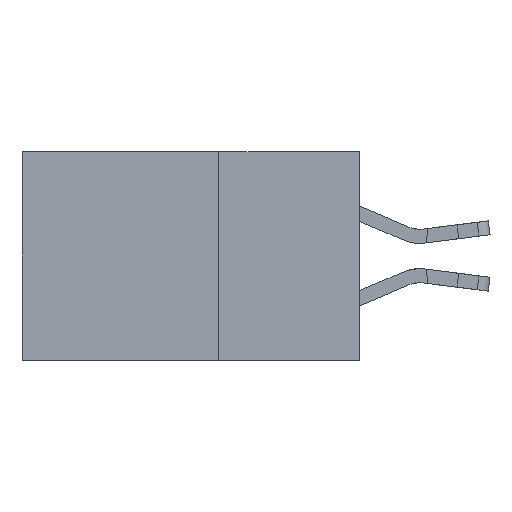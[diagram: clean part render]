
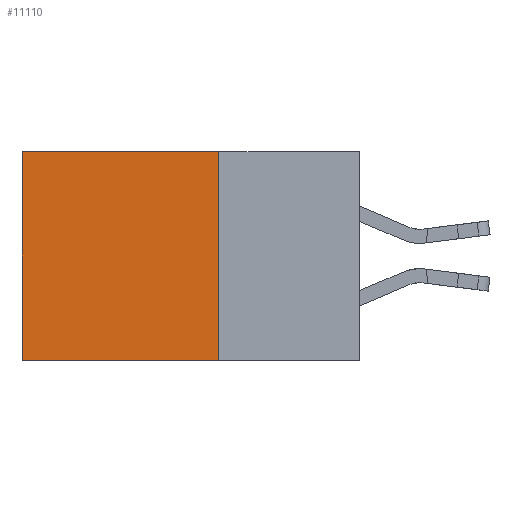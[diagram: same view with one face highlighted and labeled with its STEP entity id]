
A CAD part, left-side view. The second image highlights one B-rep face of the part: STEP entity #11110.
In plain terms, the highlighted planar face has unit normal (-1, 0, 0).
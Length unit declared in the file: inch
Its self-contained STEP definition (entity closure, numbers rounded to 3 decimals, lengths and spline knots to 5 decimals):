
#497 = CARTESIAN_POINT ( 'NONE',  ( 0.2875, 0.6, 0. ) ) ;
#4313 = LINE ( 'NONE', #4656, #7326 ) ;
#4656 = CARTESIAN_POINT ( 'NONE',  ( 0.2875, 0.25, 0. ) ) ;
#5316 = VECTOR ( 'NONE', #18281, 39.37008 ) ;
#6180 = CARTESIAN_POINT ( 'NONE',  ( 0.2875, 0.25, 0. ) ) ;
#7059 = EDGE_CURVE ( 'NONE', #25627, #17850, #20991, .T. ) ;
#7195 = DIRECTION ( 'NONE',  ( 0., 0., -1. ) ) ;
#7263 = CARTESIAN_POINT ( 'NONE',  ( 0.2875, 0.25, -0.37 ) ) ;
#7326 = VECTOR ( 'NONE', #7195, 39.37008 ) ;
#7953 = EDGE_LOOP ( 'NONE', ( #19241, #13174, #18421, #10959 ) ) ;
#8725 = DIRECTION ( 'NONE',  ( 0., 0., -1. ) ) ;
#10503 = EDGE_CURVE ( 'NONE', #16724, #11021, #24489, .T. ) ;
#10959 = ORIENTED_EDGE ( 'NONE', *, *, #10503, .T. ) ;
#11021 = VERTEX_POINT ( 'NONE', #24272 ) ;
#11110 = ADVANCED_FACE ( 'NONE', ( #14319 ), #33432, .F. ) ;
#11254 = DIRECTION ( 'NONE',  ( 1., 0., 0. ) ) ;
#11361 = DIRECTION ( 'NONE',  ( 0., 0., -1. ) ) ;
#12987 = AXIS2_PLACEMENT_3D ( 'NONE', #6180, #11254, #8725 ) ;
#13174 = ORIENTED_EDGE ( 'NONE', *, *, #7059, .F. ) ;
#14319 = FACE_OUTER_BOUND ( 'NONE', #7953, .T. ) ;
#15002 = CARTESIAN_POINT ( 'NONE',  ( 0.2875, 0.6, -0.37 ) ) ;
#16724 = VERTEX_POINT ( 'NONE', #24367 ) ;
#17850 = VERTEX_POINT ( 'NONE', #15002 ) ;
#18281 = DIRECTION ( 'NONE',  ( 0., 1., 0. ) ) ;
#18421 = ORIENTED_EDGE ( 'NONE', *, *, #34206, .F. ) ;
#19241 = ORIENTED_EDGE ( 'NONE', *, *, #19578, .T. ) ;
#19578 = EDGE_CURVE ( 'NONE', #11021, #17850, #20221, .T. ) ;
#20221 = LINE ( 'NONE', #497, #20883 ) ;
#20883 = VECTOR ( 'NONE', #11361, 39.37008 ) ;
#20991 = LINE ( 'NONE', #7263, #5316 ) ;
#21430 = CARTESIAN_POINT ( 'NONE',  ( 0.2875, 0.25, 0. ) ) ;
#24272 = CARTESIAN_POINT ( 'NONE',  ( 0.2875, 0.6, 0. ) ) ;
#24367 = CARTESIAN_POINT ( 'NONE',  ( 0.2875, 0.25, 0. ) ) ;
#24489 = LINE ( 'NONE', #21430, #25595 ) ;
#25595 = VECTOR ( 'NONE', #29898, 39.37008 ) ;
#25627 = VERTEX_POINT ( 'NONE', #35386 ) ;
#29898 = DIRECTION ( 'NONE',  ( 0., 1., 0. ) ) ;
#33432 = PLANE ( 'NONE',  #12987 ) ;
#34206 = EDGE_CURVE ( 'NONE', #16724, #25627, #4313, .T. ) ;
#35386 = CARTESIAN_POINT ( 'NONE',  ( 0.2875, 0.25, -0.37 ) ) ;
